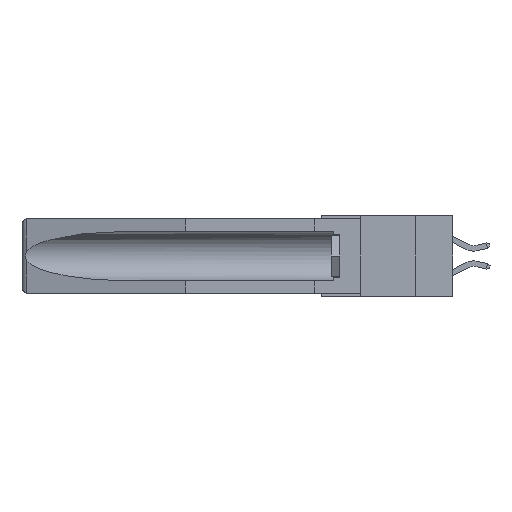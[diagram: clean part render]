
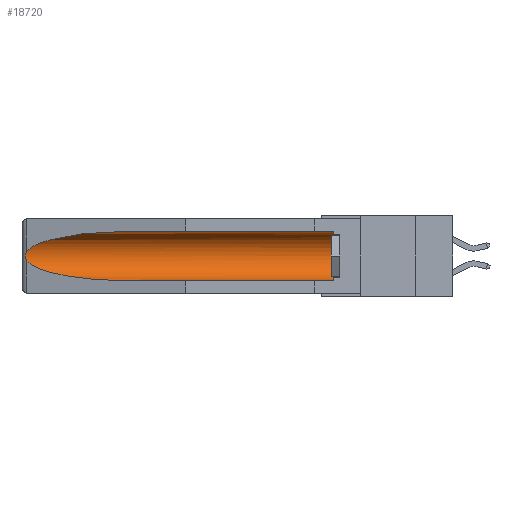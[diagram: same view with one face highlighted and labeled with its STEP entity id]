
A CAD part, left-side view. The second image highlights one B-rep face of the part: STEP entity #18720.
In plain terms, the highlighted cylindrical face has radius 2.857 mm (diameter 5.715 mm), a partial arc.
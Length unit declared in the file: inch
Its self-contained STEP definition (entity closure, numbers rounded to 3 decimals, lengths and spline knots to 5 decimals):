
#494 = B_SPLINE_CURVE_WITH_KNOTS ( 'NONE', 3,
 ( #22947, #15226, #3696, #5616, #11471, #13465, #24720, #13383, #15313, #3775 ),
 .UNSPECIFIED., .F., .F.,
 ( 4, 2, 2, 2, 4 ),
 ( 0., 0.00029, 0.00058, 0.00087, 0.00117 ),
 .UNSPECIFIED. ) ;
#595 = VECTOR ( 'NONE', #16266, 39.37008 ) ;
#1063 = DIRECTION ( 'NONE',  ( 0., 0., 1. ) ) ;
#1573 = EDGE_CURVE ( 'NONE', #4963, #22722, #5741, .T. ) ;
#1763 = EDGE_CURVE ( 'NONE', #12906, #2671, #494, .T. ) ;
#2469 = EDGE_CURVE ( 'NONE', #2671, #8432, #4213, .T. ) ;
#2671 = VERTEX_POINT ( 'NONE', #16797 ) ;
#3021 = CARTESIAN_POINT ( 'NONE',  ( 0.155, 1.07973, -0.059 ) ) ;
#3073 = EDGE_CURVE ( 'NONE', #16856, #4963, #23768, .T. ) ;
#3253 = AXIS2_PLACEMENT_3D ( 'NONE', #4168, #6186, #21663 ) ;
#3696 = CARTESIAN_POINT ( 'NONE',  ( 0.26654, 1.53092, -0.15636 ) ) ;
#3775 = CARTESIAN_POINT ( 'NONE',  ( 0.26537, 1.52718, -0.19328 ) ) ;
#4168 = CARTESIAN_POINT ( 'NONE',  ( 0.155, -0.30754, -0.1715 ) ) ;
#4213 =( BOUNDED_CURVE ( )  B_SPLINE_CURVE ( 3, ( #23989, #18333, #16458, #22303 ),
 .UNSPECIFIED., .F., .F. ) 
 B_SPLINE_CURVE_WITH_KNOTS ( ( 4, 4 ),
 ( 0.1948, 1.5708 ),
 .UNSPECIFIED. ) 
 CURVE ( )  GEOMETRIC_REPRESENTATION_ITEM ( )  RATIONAL_B_SPLINE_CURVE ( ( 1., 0.848, 0.848, 1. ) ) 
 REPRESENTATION_ITEM ( '' )  );
#4963 = VERTEX_POINT ( 'NONE', #17532 ) ;
#5029 = CARTESIAN_POINT ( 'NONE',  ( 0.26537, 1.52718, -0.14972 ) ) ;
#5525 = CYLINDRICAL_SURFACE ( 'NONE', #3253, 0.1125 ) ;
#5616 = CARTESIAN_POINT ( 'NONE',  ( 0.2673, 1.5327, -0.16383 ) ) ;
#5741 = LINE ( 'NONE', #18300, #595 ) ;
#6186 = DIRECTION ( 'NONE',  ( 0., 1., 0. ) ) ;
#6425 = FACE_OUTER_BOUND ( 'NONE', #22937, .T. ) ;
#8379 = CARTESIAN_POINT ( 'NONE',  ( 0.155, 1.07973, -0.284 ) ) ;
#8432 = VERTEX_POINT ( 'NONE', #8379 ) ;
#8602 = ORIENTED_EDGE ( 'NONE', *, *, #8989, .F. ) ;
#8989 = EDGE_CURVE ( 'NONE', #16856, #8432, #18601, .T. ) ;
#10229 =( BOUNDED_CURVE ( )  B_SPLINE_CURVE ( 3, ( #3021, #14636, #18558, #5029 ),
 .UNSPECIFIED., .F., .F. ) 
 B_SPLINE_CURVE_WITH_KNOTS ( ( 4, 4 ),
 ( 4.71239, 6.08839 ),
 .UNSPECIFIED. ) 
 CURVE ( )  GEOMETRIC_REPRESENTATION_ITEM ( )  RATIONAL_B_SPLINE_CURVE ( ( 1., 0.848, 0.848, 1. ) ) 
 REPRESENTATION_ITEM ( '' )  );
#10654 = CARTESIAN_POINT ( 'NONE',  ( 0.155, 0.126, -0.284 ) ) ;
#10918 = CARTESIAN_POINT ( 'NONE',  ( 0.155, 1.07973, -0.059 ) ) ;
#11471 = CARTESIAN_POINT ( 'NONE',  ( 0.2675, 1.53308, -0.16763 ) ) ;
#12229 = ORIENTED_EDGE ( 'NONE', *, *, #2469, .T. ) ;
#12476 = CARTESIAN_POINT ( 'NONE',  ( 0.155, 0.126, -0.1715 ) ) ;
#12658 = ORIENTED_EDGE ( 'NONE', *, *, #1573, .T. ) ;
#12906 = VERTEX_POINT ( 'NONE', #20014 ) ;
#13383 = CARTESIAN_POINT ( 'NONE',  ( 0.26655, 1.53094, -0.18657 ) ) ;
#13457 = VECTOR ( 'NONE', #14601, 39.37008 ) ;
#13465 = CARTESIAN_POINT ( 'NONE',  ( 0.2675, 1.53308, -0.17534 ) ) ;
#13562 = ORIENTED_EDGE ( 'NONE', *, *, #3073, .T. ) ;
#14601 = DIRECTION ( 'NONE',  ( 0., 1., 0. ) ) ;
#14636 = CARTESIAN_POINT ( 'NONE',  ( 0.21114, 1.30732, -0.059 ) ) ;
#15226 = CARTESIAN_POINT ( 'NONE',  ( 0.26597, 1.52961, -0.15275 ) ) ;
#15313 = CARTESIAN_POINT ( 'NONE',  ( 0.26597, 1.5296, -0.19026 ) ) ;
#16266 = DIRECTION ( 'NONE',  ( 0., 1., 0. ) ) ;
#16458 = CARTESIAN_POINT ( 'NONE',  ( 0.21114, 1.30732, -0.284 ) ) ;
#16797 = CARTESIAN_POINT ( 'NONE',  ( 0.26537, 1.52718, -0.19328 ) ) ;
#16856 = VERTEX_POINT ( 'NONE', #10654 ) ;
#16970 = ORIENTED_EDGE ( 'NONE', *, *, #19421, .T. ) ;
#17532 = CARTESIAN_POINT ( 'NONE',  ( 0.155, 0.126, -0.059 ) ) ;
#18300 = CARTESIAN_POINT ( 'NONE',  ( 0.155, -0.30754, -0.059 ) ) ;
#18333 = CARTESIAN_POINT ( 'NONE',  ( 0.25451, 1.48313, -0.24835 ) ) ;
#18558 = CARTESIAN_POINT ( 'NONE',  ( 0.25451, 1.48313, -0.09465 ) ) ;
#18601 = LINE ( 'NONE', #20393, #13457 ) ;
#18720 = ADVANCED_FACE ( 'NONE', ( #6425 ), #5525, .F. ) ;
#19421 = EDGE_CURVE ( 'NONE', #22722, #12906, #10229, .T. ) ;
#20014 = CARTESIAN_POINT ( 'NONE',  ( 0.26537, 1.52718, -0.14972 ) ) ;
#20393 = CARTESIAN_POINT ( 'NONE',  ( 0.155, -0.30754, -0.284 ) ) ;
#20427 = DIRECTION ( 'NONE',  ( 0., -1., 0. ) ) ;
#21663 = DIRECTION ( 'NONE',  ( 0., 0., 1. ) ) ;
#22303 = CARTESIAN_POINT ( 'NONE',  ( 0.155, 1.07973, -0.284 ) ) ;
#22722 = VERTEX_POINT ( 'NONE', #10918 ) ;
#22937 = EDGE_LOOP ( 'NONE', ( #16970, #23280, #12229, #8602, #13562, #12658 ) ) ;
#22947 = CARTESIAN_POINT ( 'NONE',  ( 0.26537, 1.52718, -0.14972 ) ) ;
#23139 = AXIS2_PLACEMENT_3D ( 'NONE', #12476, #20427, #1063 ) ;
#23280 = ORIENTED_EDGE ( 'NONE', *, *, #1763, .T. ) ;
#23768 = CIRCLE ( 'NONE', #23139, 0.1125 ) ;
#23989 = CARTESIAN_POINT ( 'NONE',  ( 0.26537, 1.52718, -0.19328 ) ) ;
#24720 = CARTESIAN_POINT ( 'NONE',  ( 0.2673, 1.53269, -0.17917 ) ) ;
